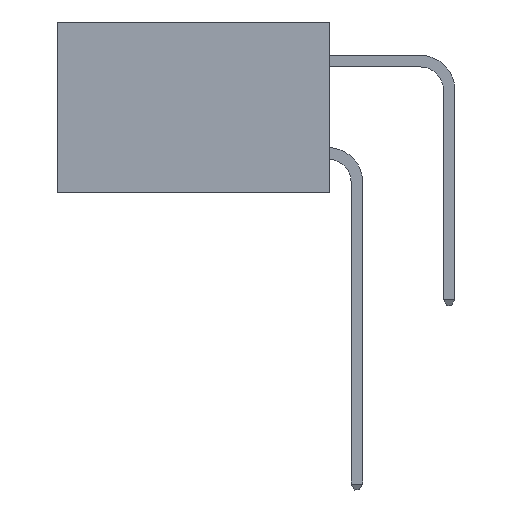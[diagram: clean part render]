
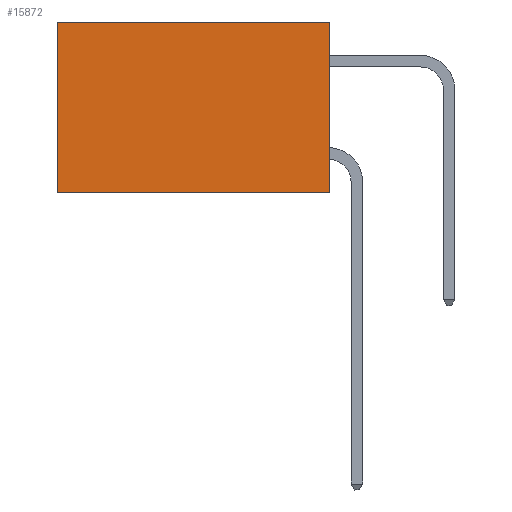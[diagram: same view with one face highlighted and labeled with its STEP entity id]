
A CAD part, left-side view. The second image highlights one B-rep face of the part: STEP entity #15872.
In plain terms, the highlighted planar face has unit normal (-1, 0, 0).
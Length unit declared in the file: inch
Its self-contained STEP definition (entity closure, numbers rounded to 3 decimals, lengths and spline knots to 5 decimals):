
#712 = LINE ( 'NONE', #5764, #12137 ) ;
#1175 = LINE ( 'NONE', #6245, #12611 ) ;
#1737 = AXIS2_PLACEMENT_3D ( 'NONE', #10786, #12260, #3314 ) ;
#3098 = CARTESIAN_POINT ( 'NONE',  ( 0.277, 0.59, -0.37 ) ) ;
#3314 = DIRECTION ( 'NONE',  ( 0., 0., -1. ) ) ;
#3325 = VERTEX_POINT ( 'NONE', #11533 ) ;
#3585 = VECTOR ( 'NONE', #15389, 39.37008 ) ;
#4807 = CARTESIAN_POINT ( 'NONE',  ( 0.277, 0., 0. ) ) ;
#4850 = ORIENTED_EDGE ( 'NONE', *, *, #11807, .T. ) ;
#5764 = CARTESIAN_POINT ( 'NONE',  ( 0.277, 0., -0.37 ) ) ;
#5897 = EDGE_CURVE ( 'NONE', #13521, #16454, #15470, .T. ) ;
#6245 = CARTESIAN_POINT ( 'NONE',  ( 0.277, 0., -0.37 ) ) ;
#6498 = CARTESIAN_POINT ( 'NONE',  ( 0.277, 0.59, -0.37 ) ) ;
#6801 = VERTEX_POINT ( 'NONE', #17159 ) ;
#6862 = EDGE_LOOP ( 'NONE', ( #15091, #18290, #11423, #4850 ) ) ;
#8829 = CARTESIAN_POINT ( 'NONE',  ( 0.277, 0.59, 0. ) ) ;
#9014 = EDGE_CURVE ( 'NONE', #3325, #6801, #1175, .T. ) ;
#9537 = EDGE_CURVE ( 'NONE', #6801, #16454, #712, .T. ) ;
#10786 = CARTESIAN_POINT ( 'NONE',  ( 0.277, 0., -0.37 ) ) ;
#11423 = ORIENTED_EDGE ( 'NONE', *, *, #9014, .F. ) ;
#11533 = CARTESIAN_POINT ( 'NONE',  ( 0.277, 0., 0. ) ) ;
#11807 = EDGE_CURVE ( 'NONE', #3325, #13521, #18712, .T. ) ;
#12137 = VECTOR ( 'NONE', #19076, 39.37008 ) ;
#12245 = DIRECTION ( 'NONE',  ( 0., 0., -1. ) ) ;
#12260 = DIRECTION ( 'NONE',  ( 1., 0., 0. ) ) ;
#12611 = VECTOR ( 'NONE', #12245, 39.37008 ) ;
#13521 = VERTEX_POINT ( 'NONE', #8829 ) ;
#13710 = PLANE ( 'NONE',  #1737 ) ;
#14930 = FACE_OUTER_BOUND ( 'NONE', #6862, .T. ) ;
#15091 = ORIENTED_EDGE ( 'NONE', *, *, #5897, .T. ) ;
#15160 = DIRECTION ( 'NONE',  ( 0., 1., 0. ) ) ;
#15389 = DIRECTION ( 'NONE',  ( 0., 0., -1. ) ) ;
#15470 = LINE ( 'NONE', #6498, #3585 ) ;
#15747 = VECTOR ( 'NONE', #15160, 39.37008 ) ;
#15872 = ADVANCED_FACE ( 'NONE', ( #14930 ), #13710, .F. ) ;
#16454 = VERTEX_POINT ( 'NONE', #3098 ) ;
#17159 = CARTESIAN_POINT ( 'NONE',  ( 0.277, 0., -0.37 ) ) ;
#18290 = ORIENTED_EDGE ( 'NONE', *, *, #9537, .F. ) ;
#18712 = LINE ( 'NONE', #4807, #15747 ) ;
#19076 = DIRECTION ( 'NONE',  ( 0., 1., 0. ) ) ;
